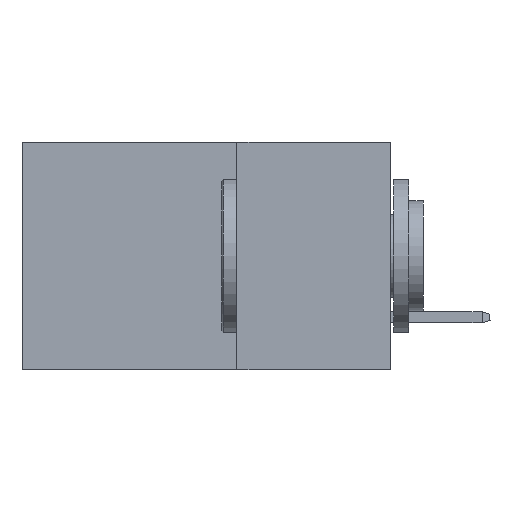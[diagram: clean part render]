
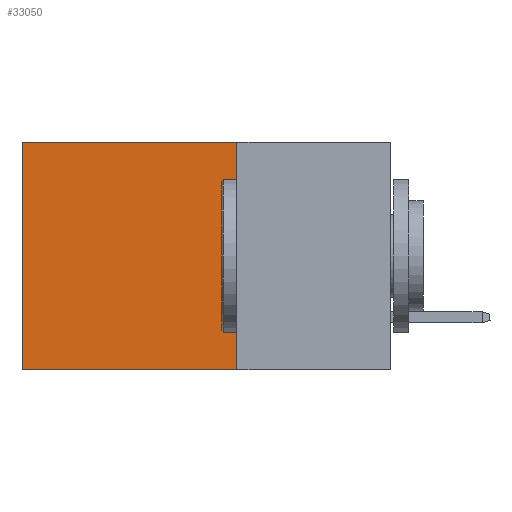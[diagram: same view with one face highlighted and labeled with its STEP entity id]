
A CAD part, left-side view. The second image highlights one B-rep face of the part: STEP entity #33050.
In plain terms, the highlighted planar face has unit normal (-1, 0, 0).
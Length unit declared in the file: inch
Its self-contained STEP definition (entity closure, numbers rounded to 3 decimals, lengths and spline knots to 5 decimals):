
#225 = CARTESIAN_POINT ( 'NONE',  ( 0.2875, 0.6, 0. ) ) ;
#388 = VECTOR ( 'NONE', #10073, 39.37008 ) ;
#1345 = VERTEX_POINT ( 'NONE', #23983 ) ;
#2535 = EDGE_CURVE ( 'NONE', #16541, #24190, #10636, .T. ) ;
#2985 = CARTESIAN_POINT ( 'NONE',  ( 0.2875, 0.25, 0. ) ) ;
#5262 = FACE_OUTER_BOUND ( 'NONE', #10445, .T. ) ;
#6919 = ORIENTED_EDGE ( 'NONE', *, *, #22001, .F. ) ;
#9494 = DIRECTION ( 'NONE',  ( 0., 0., -1. ) ) ;
#10073 = DIRECTION ( 'NONE',  ( 0., 0., -1. ) ) ;
#10380 = CARTESIAN_POINT ( 'NONE',  ( 0.2875, 0.25, 0. ) ) ;
#10445 = EDGE_LOOP ( 'NONE', ( #12919, #6919, #13195, #28104 ) ) ;
#10636 = LINE ( 'NONE', #15365, #388 ) ;
#11350 = DIRECTION ( 'NONE',  ( 0., 1., 0. ) ) ;
#12244 = DIRECTION ( 'NONE',  ( 1., 0., 0. ) ) ;
#12919 = ORIENTED_EDGE ( 'NONE', *, *, #15047, .T. ) ;
#13041 = CARTESIAN_POINT ( 'NONE',  ( 0.2875, 0.25, -0.37 ) ) ;
#13195 = ORIENTED_EDGE ( 'NONE', *, *, #2535, .F. ) ;
#13937 = EDGE_CURVE ( 'NONE', #16541, #22709, #19679, .T. ) ;
#14554 = LINE ( 'NONE', #13041, #23549 ) ;
#15047 = EDGE_CURVE ( 'NONE', #22709, #1345, #29383, .T. ) ;
#15365 = CARTESIAN_POINT ( 'NONE',  ( 0.2875, 0.25, 0. ) ) ;
#16436 = CARTESIAN_POINT ( 'NONE',  ( 0.2875, 0.25, -0.37 ) ) ;
#16541 = VERTEX_POINT ( 'NONE', #10380 ) ;
#19679 = LINE ( 'NONE', #2985, #33317 ) ;
#22001 = EDGE_CURVE ( 'NONE', #24190, #1345, #14554, .T. ) ;
#22709 = VERTEX_POINT ( 'NONE', #27591 ) ;
#23549 = VECTOR ( 'NONE', #29174, 39.37008 ) ;
#23983 = CARTESIAN_POINT ( 'NONE',  ( 0.2875, 0.6, -0.37 ) ) ;
#24190 = VERTEX_POINT ( 'NONE', #16436 ) ;
#27591 = CARTESIAN_POINT ( 'NONE',  ( 0.2875, 0.6, 0. ) ) ;
#28104 = ORIENTED_EDGE ( 'NONE', *, *, #13937, .T. ) ;
#28126 = VECTOR ( 'NONE', #33221, 39.37008 ) ;
#28530 = CARTESIAN_POINT ( 'NONE',  ( 0.2875, 0.25, 0. ) ) ;
#28982 = AXIS2_PLACEMENT_3D ( 'NONE', #28530, #12244, #9494 ) ;
#29174 = DIRECTION ( 'NONE',  ( 0., 1., 0. ) ) ;
#29383 = LINE ( 'NONE', #225, #28126 ) ;
#31477 = PLANE ( 'NONE',  #28982 ) ;
#33050 = ADVANCED_FACE ( 'NONE', ( #5262 ), #31477, .F. ) ;
#33221 = DIRECTION ( 'NONE',  ( 0., 0., -1. ) ) ;
#33317 = VECTOR ( 'NONE', #11350, 39.37008 ) ;
